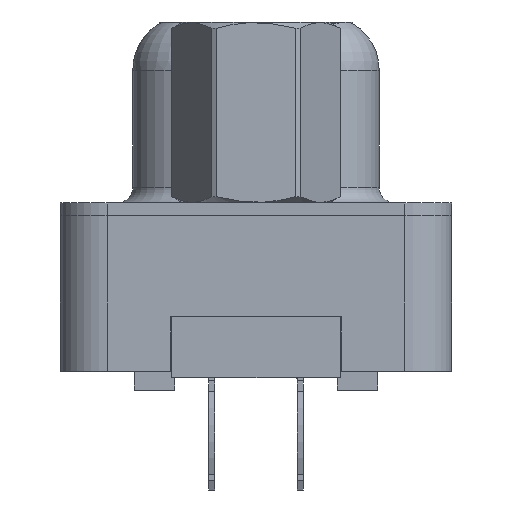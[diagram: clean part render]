
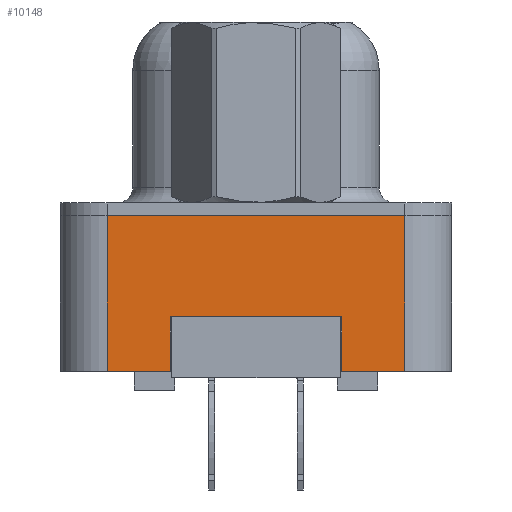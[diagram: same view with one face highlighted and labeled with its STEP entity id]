
A CAD part, left-side view. The second image highlights one B-rep face of the part: STEP entity #10148.
In plain terms, the highlighted planar face has unit normal (-1, 0, 0).
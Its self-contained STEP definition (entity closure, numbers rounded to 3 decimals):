
#434 = CARTESIAN_POINT ( 'NONE',  ( -2.995, 4.775, -5. ) ) ;
#794 = EDGE_CURVE ( 'NONE', #6836, #18858, #15874, .T. ) ;
#1702 = VECTOR ( 'NONE', #18666, 1000. ) ;
#2070 = CARTESIAN_POINT ( 'NONE',  ( -2.995, 2.75, -3.25 ) ) ;
#2299 = CARTESIAN_POINT ( 'NONE',  ( -2.995, 2.75, -3.25 ) ) ;
#2387 = VECTOR ( 'NONE', #17114, 1000. ) ;
#2792 = VECTOR ( 'NONE', #11134, 1000. ) ;
#3063 = EDGE_CURVE ( 'NONE', #18858, #17267, #14229, .T. ) ;
#3272 = VECTOR ( 'NONE', #18397, 1000. ) ;
#3428 = CARTESIAN_POINT ( 'NONE',  ( -2.995, -4.775, -5. ) ) ;
#3702 = VERTEX_POINT ( 'NONE', #2299 ) ;
#3933 = ORIENTED_EDGE ( 'NONE', *, *, #9493, .F. ) ;
#3998 = CARTESIAN_POINT ( 'NONE',  ( -2.995, 2.75, -5. ) ) ;
#4151 = VERTEX_POINT ( 'NONE', #5507 ) ;
#4440 = EDGE_LOOP ( 'NONE', ( #21237, #18091, #5127, #8446, #17368, #8855, #24114, #3933 ) ) ;
#4586 = LINE ( 'NONE', #21087, #1702 ) ;
#4826 = VECTOR ( 'NONE', #6119, 1000. ) ;
#4851 = VECTOR ( 'NONE', #10189, 1000. ) ;
#5127 = ORIENTED_EDGE ( 'NONE', *, *, #3063, .T. ) ;
#5148 = CARTESIAN_POINT ( 'NONE',  ( -2.995, -2.75, -3.25 ) ) ;
#5446 = LINE ( 'NONE', #25831, #2387 ) ;
#5507 = CARTESIAN_POINT ( 'NONE',  ( -2.995, 4.775, 0. ) ) ;
#5725 = CARTESIAN_POINT ( 'NONE',  ( -2.995, -4.775, -5. ) ) ;
#5824 = DIRECTION ( 'NONE',  ( 0., -1., 0. ) ) ;
#6119 = DIRECTION ( 'NONE',  ( 0., 0., -1. ) ) ;
#6836 = VERTEX_POINT ( 'NONE', #19339 ) ;
#8185 = VERTEX_POINT ( 'NONE', #434 ) ;
#8446 = ORIENTED_EDGE ( 'NONE', *, *, #16342, .F. ) ;
#8687 = EDGE_CURVE ( 'NONE', #8185, #12898, #25843, .T. ) ;
#8693 = LINE ( 'NONE', #12829, #4851 ) ;
#8855 = ORIENTED_EDGE ( 'NONE', *, *, #8687, .T. ) ;
#9493 = EDGE_CURVE ( 'NONE', #21917, #3702, #4586, .T. ) ;
#9946 = CARTESIAN_POINT ( 'NONE',  ( -2.995, -4.775, -5. ) ) ;
#10148 = ADVANCED_FACE ( 'NONE', ( #24109 ), #23571, .T. ) ;
#10189 = DIRECTION ( 'NONE',  ( 0., -1., 0. ) ) ;
#10469 = CARTESIAN_POINT ( 'NONE',  ( -2.995, -4.775, -5. ) ) ;
#11134 = DIRECTION ( 'NONE',  ( 0., 0., 1. ) ) ;
#11197 = VECTOR ( 'NONE', #5824, 1000. ) ;
#11887 = LINE ( 'NONE', #2070, #4826 ) ;
#12421 = AXIS2_PLACEMENT_3D ( 'NONE', #5725, #13896, #26239 ) ;
#12574 = CARTESIAN_POINT ( 'NONE',  ( -2.995, -4.775, 0. ) ) ;
#12829 = CARTESIAN_POINT ( 'NONE',  ( -2.995, -4.775, 0. ) ) ;
#12898 = VERTEX_POINT ( 'NONE', #3998 ) ;
#13795 = EDGE_CURVE ( 'NONE', #3702, #12898, #11887, .T. ) ;
#13864 = CARTESIAN_POINT ( 'NONE',  ( -2.995, -4.775, -5. ) ) ;
#13896 = DIRECTION ( 'NONE',  ( -1., 0., 0. ) ) ;
#14229 = LINE ( 'NONE', #10469, #3272 ) ;
#15874 = LINE ( 'NONE', #13864, #11197 ) ;
#16342 = EDGE_CURVE ( 'NONE', #4151, #17267, #8693, .T. ) ;
#17114 = DIRECTION ( 'NONE',  ( 0., 0., -1. ) ) ;
#17267 = VERTEX_POINT ( 'NONE', #12574 ) ;
#17368 = ORIENTED_EDGE ( 'NONE', *, *, #24182, .F. ) ;
#17436 = LINE ( 'NONE', #25890, #2792 ) ;
#18091 = ORIENTED_EDGE ( 'NONE', *, *, #794, .T. ) ;
#18397 = DIRECTION ( 'NONE',  ( 0., 0., 1. ) ) ;
#18666 = DIRECTION ( 'NONE',  ( 0., 1., 0. ) ) ;
#18858 = VERTEX_POINT ( 'NONE', #9946 ) ;
#19339 = CARTESIAN_POINT ( 'NONE',  ( -2.995, -2.75, -5. ) ) ;
#19680 = DIRECTION ( 'NONE',  ( 0., -1., 0. ) ) ;
#21087 = CARTESIAN_POINT ( 'NONE',  ( -2.995, 2.75, -3.25 ) ) ;
#21237 = ORIENTED_EDGE ( 'NONE', *, *, #25970, .T. ) ;
#21917 = VERTEX_POINT ( 'NONE', #5148 ) ;
#23571 = PLANE ( 'NONE',  #12421 ) ;
#24109 = FACE_OUTER_BOUND ( 'NONE', #4440, .T. ) ;
#24114 = ORIENTED_EDGE ( 'NONE', *, *, #13795, .F. ) ;
#24182 = EDGE_CURVE ( 'NONE', #8185, #4151, #17436, .T. ) ;
#25225 = VECTOR ( 'NONE', #19680, 1000. ) ;
#25831 = CARTESIAN_POINT ( 'NONE',  ( -2.995, -2.75, -3.25 ) ) ;
#25843 = LINE ( 'NONE', #3428, #25225 ) ;
#25890 = CARTESIAN_POINT ( 'NONE',  ( -2.995, 4.775, -5. ) ) ;
#25970 = EDGE_CURVE ( 'NONE', #21917, #6836, #5446, .T. ) ;
#26239 = DIRECTION ( 'NONE',  ( 0., 0., 1. ) ) ;
